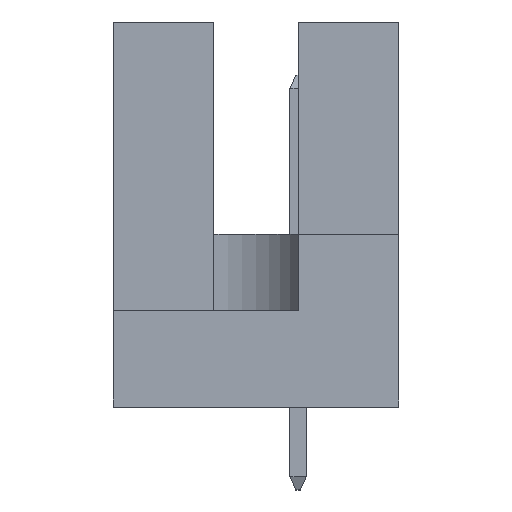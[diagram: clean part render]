
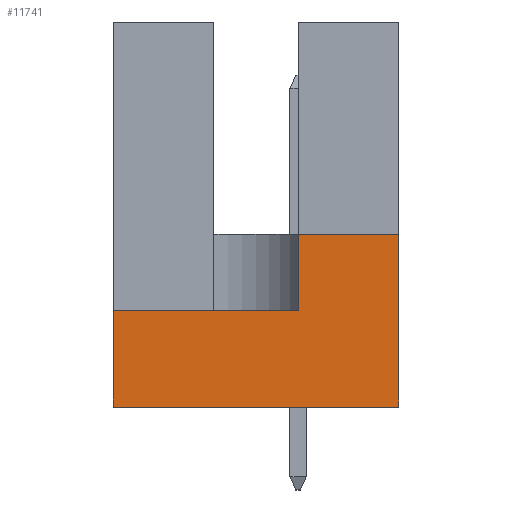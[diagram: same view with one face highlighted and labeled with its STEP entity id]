
A CAD part, left-side view. The second image highlights one B-rep face of the part: STEP entity #11741.
In plain terms, the highlighted planar face has unit normal (-1, 0, 0).
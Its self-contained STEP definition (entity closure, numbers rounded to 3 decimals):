
#256 = LINE ( 'NONE', #11119, #4543 ) ;
#787 = LINE ( 'NONE', #4509, #7404 ) ;
#947 = CARTESIAN_POINT ( 'NONE',  ( -47.5, -1.27, 5.2 ) ) ;
#994 = CARTESIAN_POINT ( 'NONE',  ( -47.5, 4.3, 2.9 ) ) ;
#1336 = CARTESIAN_POINT ( 'NONE',  ( -47.5, 4.3, 0. ) ) ;
#1352 = VERTEX_POINT ( 'NONE', #994 ) ;
#1456 = ORIENTED_EDGE ( 'NONE', *, *, #10486, .F. ) ;
#2034 = EDGE_CURVE ( 'NONE', #1352, #9382, #256, .T. ) ;
#2245 = LINE ( 'NONE', #1336, #10735 ) ;
#2392 = AXIS2_PLACEMENT_3D ( 'NONE', #6450, #8196, #7425 ) ;
#2507 = CARTESIAN_POINT ( 'NONE',  ( -47.5, 4.3, 0. ) ) ;
#2508 = VECTOR ( 'NONE', #3615, 1000. ) ;
#2618 = VECTOR ( 'NONE', #10443, 1000. ) ;
#2806 = PLANE ( 'NONE',  #2392 ) ;
#2948 = CARTESIAN_POINT ( 'NONE',  ( -47.5, -4.3, 5.2 ) ) ;
#3093 = EDGE_CURVE ( 'NONE', #5332, #4129, #9138, .T. ) ;
#3354 = LINE ( 'NONE', #10607, #7297 ) ;
#3615 = DIRECTION ( 'NONE',  ( 0., 0., -1. ) ) ;
#3636 = VERTEX_POINT ( 'NONE', #9474 ) ;
#3878 = EDGE_LOOP ( 'NONE', ( #11083, #6504, #4250, #4699, #7875, #1456 ) ) ;
#4129 = VERTEX_POINT ( 'NONE', #11372 ) ;
#4250 = ORIENTED_EDGE ( 'NONE', *, *, #7098, .T. ) ;
#4509 = CARTESIAN_POINT ( 'NONE',  ( -47.5, 4.3, 2.9 ) ) ;
#4543 = VECTOR ( 'NONE', #6557, 1000. ) ;
#4699 = ORIENTED_EDGE ( 'NONE', *, *, #2034, .T. ) ;
#4999 = DIRECTION ( 'NONE',  ( 0., -1., 0. ) ) ;
#5186 = EDGE_CURVE ( 'NONE', #5332, #9123, #5826, .T. ) ;
#5332 = VERTEX_POINT ( 'NONE', #947 ) ;
#5826 = LINE ( 'NONE', #6781, #2618 ) ;
#5939 = DIRECTION ( 'NONE',  ( 0., 0., -1. ) ) ;
#6450 = CARTESIAN_POINT ( 'NONE',  ( -47.5, 4.3, 11.6 ) ) ;
#6504 = ORIENTED_EDGE ( 'NONE', *, *, #3093, .T. ) ;
#6557 = DIRECTION ( 'NONE',  ( 0., 0., -1. ) ) ;
#6781 = CARTESIAN_POINT ( 'NONE',  ( -47.5, 4.3, 5.2 ) ) ;
#7098 = EDGE_CURVE ( 'NONE', #4129, #1352, #787, .T. ) ;
#7209 = DIRECTION ( 'NONE',  ( 0., 1., 0. ) ) ;
#7297 = VECTOR ( 'NONE', #5939, 1000. ) ;
#7358 = FACE_OUTER_BOUND ( 'NONE', #3878, .T. ) ;
#7404 = VECTOR ( 'NONE', #7209, 1000. ) ;
#7425 = DIRECTION ( 'NONE',  ( 0., 0., -1. ) ) ;
#7875 = ORIENTED_EDGE ( 'NONE', *, *, #10020, .T. ) ;
#8179 = CARTESIAN_POINT ( 'NONE',  ( -47.5, -1.27, 19.02 ) ) ;
#8196 = DIRECTION ( 'NONE',  ( 1., 0., 0. ) ) ;
#9123 = VERTEX_POINT ( 'NONE', #2948 ) ;
#9138 = LINE ( 'NONE', #8179, #2508 ) ;
#9382 = VERTEX_POINT ( 'NONE', #2507 ) ;
#9474 = CARTESIAN_POINT ( 'NONE',  ( -47.5, -4.3, 0. ) ) ;
#10020 = EDGE_CURVE ( 'NONE', #9382, #3636, #2245, .T. ) ;
#10443 = DIRECTION ( 'NONE',  ( 0., -1., 0. ) ) ;
#10486 = EDGE_CURVE ( 'NONE', #9123, #3636, #3354, .T. ) ;
#10607 = CARTESIAN_POINT ( 'NONE',  ( -47.5, -4.3, 11.6 ) ) ;
#10735 = VECTOR ( 'NONE', #4999, 1000. ) ;
#11083 = ORIENTED_EDGE ( 'NONE', *, *, #5186, .F. ) ;
#11119 = CARTESIAN_POINT ( 'NONE',  ( -47.5, 4.3, 11.6 ) ) ;
#11372 = CARTESIAN_POINT ( 'NONE',  ( -47.5, -1.27, 2.9 ) ) ;
#11741 = ADVANCED_FACE ( 'NONE', ( #7358 ), #2806, .F. ) ;
